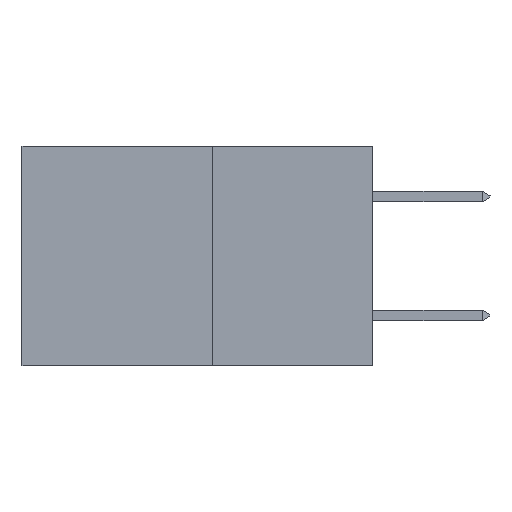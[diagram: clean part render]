
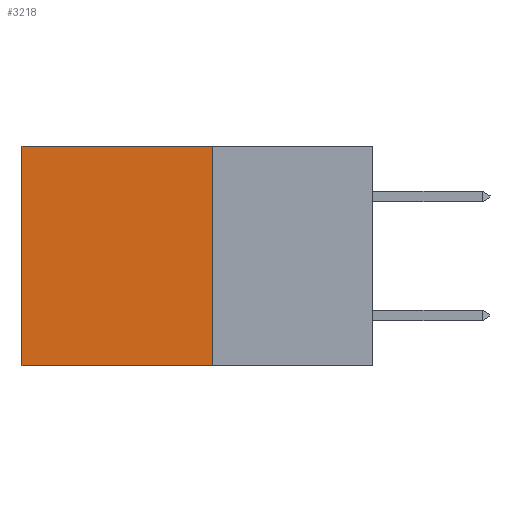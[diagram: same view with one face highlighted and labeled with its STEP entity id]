
A CAD part, left-side view. The second image highlights one B-rep face of the part: STEP entity #3218.
In plain terms, the highlighted planar face has unit normal (-1, 0, 0).
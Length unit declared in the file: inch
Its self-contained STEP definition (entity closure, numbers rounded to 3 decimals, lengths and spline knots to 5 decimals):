
#172 = CARTESIAN_POINT ( 'NONE',  ( 0.277, 0.59, -0.37 ) ) ;
#255 = ORIENTED_EDGE ( 'NONE', *, *, #339, .F. ) ;
#339 = EDGE_CURVE ( 'NONE', #5968, #2629, #3181, .T. ) ;
#387 = DIRECTION ( 'NONE',  ( 0., 0., -1. ) ) ;
#480 = CARTESIAN_POINT ( 'NONE',  ( 0.277, 0.27, -0.37 ) ) ;
#1182 = VERTEX_POINT ( 'NONE', #5237 ) ;
#1185 = DIRECTION ( 'NONE',  ( 0., 0., -1. ) ) ;
#1202 = ORIENTED_EDGE ( 'NONE', *, *, #7210, .F. ) ;
#1249 = DIRECTION ( 'NONE',  ( 0., 1., 0. ) ) ;
#1727 = VECTOR ( 'NONE', #387, 39.37008 ) ;
#1844 = LINE ( 'NONE', #172, #6134 ) ;
#2103 = CARTESIAN_POINT ( 'NONE',  ( 0.277, 0.27, 0. ) ) ;
#2239 = AXIS2_PLACEMENT_3D ( 'NONE', #10090, #9961, #9958 ) ;
#2526 = VERTEX_POINT ( 'NONE', #10949 ) ;
#2629 = VERTEX_POINT ( 'NONE', #4887 ) ;
#3181 = LINE ( 'NONE', #10686, #7423 ) ;
#3218 = ADVANCED_FACE ( 'NONE', ( #3696 ), #9968, .F. ) ;
#3696 = FACE_OUTER_BOUND ( 'NONE', #11083, .T. ) ;
#4887 = CARTESIAN_POINT ( 'NONE',  ( 0.277, 0.59, -0.37 ) ) ;
#5237 = CARTESIAN_POINT ( 'NONE',  ( 0.277, 0.59, 0. ) ) ;
#5794 = ORIENTED_EDGE ( 'NONE', *, *, #9575, .T. ) ;
#5968 = VERTEX_POINT ( 'NONE', #6343 ) ;
#6133 = VECTOR ( 'NONE', #1249, 39.37008 ) ;
#6134 = VECTOR ( 'NONE', #1185, 39.37008 ) ;
#6278 = LINE ( 'NONE', #480, #1727 ) ;
#6343 = CARTESIAN_POINT ( 'NONE',  ( 0.277, 0.27, -0.37 ) ) ;
#7210 = EDGE_CURVE ( 'NONE', #2526, #5968, #6278, .T. ) ;
#7423 = VECTOR ( 'NONE', #10898, 39.37008 ) ;
#8058 = EDGE_CURVE ( 'NONE', #1182, #2629, #1844, .T. ) ;
#8386 = LINE ( 'NONE', #2103, #6133 ) ;
#8982 = ORIENTED_EDGE ( 'NONE', *, *, #8058, .T. ) ;
#9575 = EDGE_CURVE ( 'NONE', #2526, #1182, #8386, .T. ) ;
#9958 = DIRECTION ( 'NONE',  ( 0., 0., -1. ) ) ;
#9961 = DIRECTION ( 'NONE',  ( 1., 0., 0. ) ) ;
#9968 = PLANE ( 'NONE',  #2239 ) ;
#10090 = CARTESIAN_POINT ( 'NONE',  ( 0.277, 0.27, -0.37 ) ) ;
#10686 = CARTESIAN_POINT ( 'NONE',  ( 0.277, 0.27, -0.37 ) ) ;
#10898 = DIRECTION ( 'NONE',  ( 0., 1., 0. ) ) ;
#10949 = CARTESIAN_POINT ( 'NONE',  ( 0.277, 0.27, 0. ) ) ;
#11083 = EDGE_LOOP ( 'NONE', ( #8982, #255, #1202, #5794 ) ) ;
